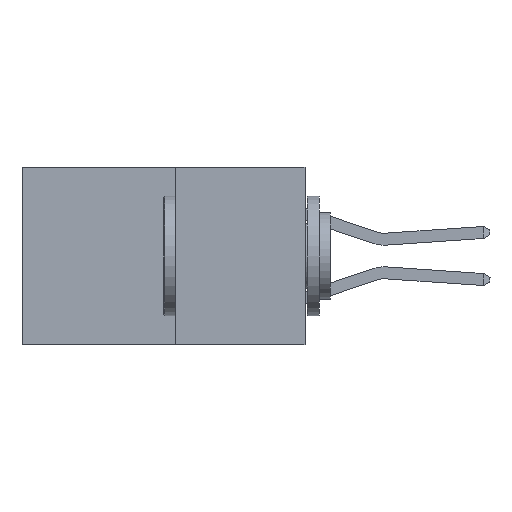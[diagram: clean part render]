
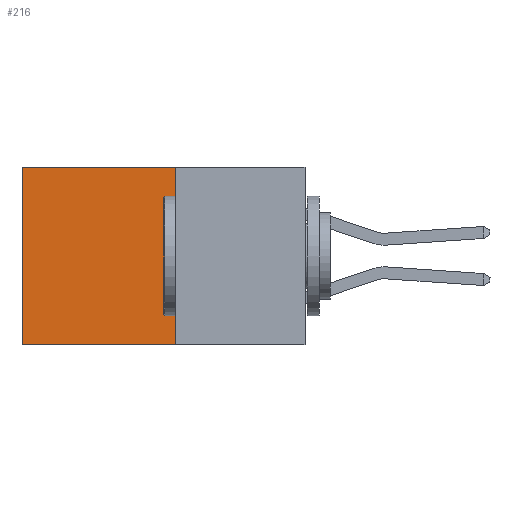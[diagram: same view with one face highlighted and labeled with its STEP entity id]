
A CAD part, left-side view. The second image highlights one B-rep face of the part: STEP entity #216.
In plain terms, the highlighted planar face has unit normal (-1, 0, 0).
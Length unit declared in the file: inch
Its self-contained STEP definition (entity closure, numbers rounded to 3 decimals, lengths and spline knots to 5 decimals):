
#90 = CARTESIAN_POINT ( 'NONE',  ( 0.277, 0.59, 0. ) ) ;
#140 = DIRECTION ( 'NONE',  ( 0., 0., -1. ) ) ;
#216 = ADVANCED_FACE ( 'NONE', ( #6815 ), #11094, .F. ) ;
#254 = VERTEX_POINT ( 'NONE', #10043 ) ;
#902 = VECTOR ( 'NONE', #8492, 39.37008 ) ;
#930 = CARTESIAN_POINT ( 'NONE',  ( 0.277, 0.59, -0.37 ) ) ;
#1399 = EDGE_CURVE ( 'NONE', #8219, #2201, #11017, .T. ) ;
#1557 = EDGE_CURVE ( 'NONE', #254, #8219, #9092, .T. ) ;
#1831 = DIRECTION ( 'NONE',  ( 0., 1., 0. ) ) ;
#1844 = CARTESIAN_POINT ( 'NONE',  ( 0.277, 0.27, 0. ) ) ;
#1935 = EDGE_CURVE ( 'NONE', #2881, #2201, #6630, .T. ) ;
#2201 = VERTEX_POINT ( 'NONE', #930 ) ;
#2248 = VECTOR ( 'NONE', #1831, 39.37008 ) ;
#2881 = VERTEX_POINT ( 'NONE', #90 ) ;
#2967 = CARTESIAN_POINT ( 'NONE',  ( 0.277, 0.59, -0.37 ) ) ;
#3074 = EDGE_LOOP ( 'NONE', ( #6041, #3728, #6326, #8757 ) ) ;
#3514 = DIRECTION ( 'NONE',  ( 1., 0., 0. ) ) ;
#3633 = CARTESIAN_POINT ( 'NONE',  ( 0.277, 0.27, -0.37 ) ) ;
#3728 = ORIENTED_EDGE ( 'NONE', *, *, #1399, .F. ) ;
#4857 = EDGE_CURVE ( 'NONE', #254, #2881, #7161, .T. ) ;
#4979 = AXIS2_PLACEMENT_3D ( 'NONE', #3633, #3514, #7681 ) ;
#6041 = ORIENTED_EDGE ( 'NONE', *, *, #1935, .T. ) ;
#6181 = DIRECTION ( 'NONE',  ( 0., 0., -1. ) ) ;
#6326 = ORIENTED_EDGE ( 'NONE', *, *, #1557, .F. ) ;
#6538 = CARTESIAN_POINT ( 'NONE',  ( 0.277, 0.27, -0.37 ) ) ;
#6630 = LINE ( 'NONE', #2967, #9080 ) ;
#6815 = FACE_OUTER_BOUND ( 'NONE', #3074, .T. ) ;
#7161 = LINE ( 'NONE', #1844, #2248 ) ;
#7313 = CARTESIAN_POINT ( 'NONE',  ( 0.277, 0.27, -0.37 ) ) ;
#7681 = DIRECTION ( 'NONE',  ( 0., 0., -1. ) ) ;
#8219 = VERTEX_POINT ( 'NONE', #7313 ) ;
#8492 = DIRECTION ( 'NONE',  ( 0., 1., 0. ) ) ;
#8522 = VECTOR ( 'NONE', #6181, 39.37008 ) ;
#8757 = ORIENTED_EDGE ( 'NONE', *, *, #4857, .T. ) ;
#9080 = VECTOR ( 'NONE', #140, 39.37008 ) ;
#9092 = LINE ( 'NONE', #6538, #8522 ) ;
#9172 = CARTESIAN_POINT ( 'NONE',  ( 0.277, 0.27, -0.37 ) ) ;
#10043 = CARTESIAN_POINT ( 'NONE',  ( 0.277, 0.27, 0. ) ) ;
#11017 = LINE ( 'NONE', #9172, #902 ) ;
#11094 = PLANE ( 'NONE',  #4979 ) ;
